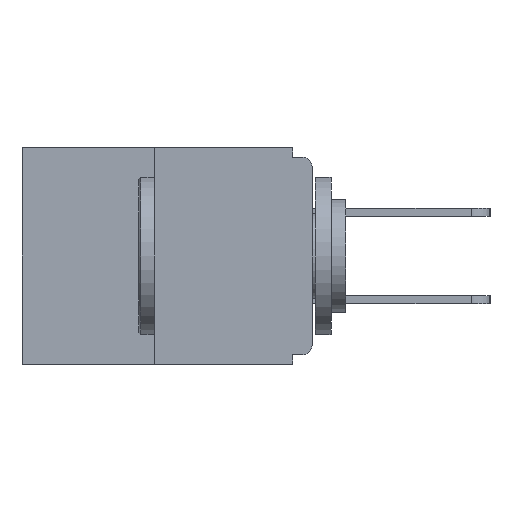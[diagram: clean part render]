
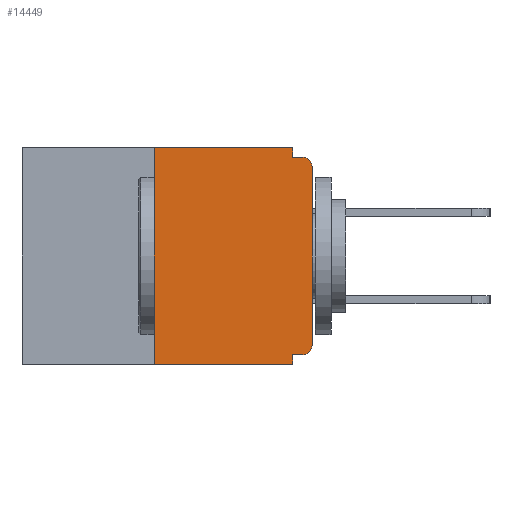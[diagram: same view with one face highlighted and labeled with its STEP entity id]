
A CAD part, left-side view. The second image highlights one B-rep face of the part: STEP entity #14449.
In plain terms, the highlighted planar face has unit normal (-1, 0, 0).
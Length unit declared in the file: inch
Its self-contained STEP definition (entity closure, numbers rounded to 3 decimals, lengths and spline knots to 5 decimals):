
#1213 = DIRECTION ( 'NONE',  ( 0., 0., -1. ) ) ;
#1293 = ORIENTED_EDGE ( 'NONE', *, *, #26827, .T. ) ;
#1649 = LINE ( 'NONE', #18349, #19434 ) ;
#1772 = CARTESIAN_POINT ( 'NONE',  ( 0., 0., -0.313 ) ) ;
#2065 = ORIENTED_EDGE ( 'NONE', *, *, #16569, .T. ) ;
#2437 = VERTEX_POINT ( 'NONE', #18296 ) ;
#2688 = VERTEX_POINT ( 'NONE', #1772 ) ;
#3040 = ORIENTED_EDGE ( 'NONE', *, *, #24897, .T. ) ;
#3080 = CARTESIAN_POINT ( 'NONE',  ( 0., 0., -0.015 ) ) ;
#3087 = ORIENTED_EDGE ( 'NONE', *, *, #24577, .F. ) ;
#3445 = VERTEX_POINT ( 'NONE', #12767 ) ;
#3453 = DIRECTION ( 'NONE',  ( 0., -1., 0. ) ) ;
#4231 = CARTESIAN_POINT ( 'NONE',  ( 0., 0.25, 0. ) ) ;
#4738 = CIRCLE ( 'NONE', #22174, 0.015 ) ;
#5225 = VECTOR ( 'NONE', #21056, 39.37008 ) ;
#5918 = DIRECTION ( 'NONE',  ( 0., 0., 1. ) ) ;
#6887 = DIRECTION ( 'NONE',  ( 0., 0., -1. ) ) ;
#7381 = AXIS2_PLACEMENT_3D ( 'NONE', #15510, #19994, #6887 ) ;
#7421 = CARTESIAN_POINT ( 'NONE',  ( 0., 0.25, -0.343 ) ) ;
#7427 = LINE ( 'NONE', #14130, #16721 ) ;
#7501 = EDGE_CURVE ( 'NONE', #11751, #8629, #21287, .T. ) ;
#7708 = DIRECTION ( 'NONE',  ( 0., 1., 0. ) ) ;
#8007 = EDGE_CURVE ( 'NONE', #20394, #11751, #28143, .T. ) ;
#8028 = VERTEX_POINT ( 'NONE', #23538 ) ;
#8281 = LINE ( 'NONE', #24374, #10684 ) ;
#8629 = VERTEX_POINT ( 'NONE', #19067 ) ;
#8631 = CARTESIAN_POINT ( 'NONE',  ( 0., 0.031, 0. ) ) ;
#9191 = VERTEX_POINT ( 'NONE', #15199 ) ;
#9942 = EDGE_CURVE ( 'NONE', #8028, #9191, #1649, .T. ) ;
#10440 = DIRECTION ( 'NONE',  ( 0., 0., -1. ) ) ;
#10616 = FACE_OUTER_BOUND ( 'NONE', #19601, .T. ) ;
#10684 = VECTOR ( 'NONE', #17773, 39.37008 ) ;
#11025 = ORIENTED_EDGE ( 'NONE', *, *, #12211, .F. ) ;
#11477 = EDGE_CURVE ( 'NONE', #2437, #20394, #26867, .T. ) ;
#11751 = VERTEX_POINT ( 'NONE', #15327 ) ;
#12211 = EDGE_CURVE ( 'NONE', #14949, #2437, #26182, .T. ) ;
#12767 = CARTESIAN_POINT ( 'NONE',  ( 0., 0., -0.03 ) ) ;
#13080 = LINE ( 'NONE', #20679, #15150 ) ;
#13696 = AXIS2_PLACEMENT_3D ( 'NONE', #27669, #25569, #10440 ) ;
#14022 = VECTOR ( 'NONE', #15320, 39.37008 ) ;
#14130 = CARTESIAN_POINT ( 'NONE',  ( 0., 0., 0. ) ) ;
#14449 = ADVANCED_FACE ( 'NONE', ( #10616 ), #25957, .F. ) ;
#14620 = VERTEX_POINT ( 'NONE', #17353 ) ;
#14949 = VERTEX_POINT ( 'NONE', #7421 ) ;
#15150 = VECTOR ( 'NONE', #1213, 39.37008 ) ;
#15199 = CARTESIAN_POINT ( 'NONE',  ( 0., 0.031, -0.328 ) ) ;
#15320 = DIRECTION ( 'NONE',  ( 0., 0., -1. ) ) ;
#15327 = CARTESIAN_POINT ( 'NONE',  ( 0., 0.031, -0.015 ) ) ;
#15460 = VECTOR ( 'NONE', #24614, 39.37008 ) ;
#15510 = CARTESIAN_POINT ( 'NONE',  ( 0., 0.015, -0.313 ) ) ;
#16569 = EDGE_CURVE ( 'NONE', #2688, #3445, #7427, .T. ) ;
#16721 = VECTOR ( 'NONE', #5918, 39.37008 ) ;
#16886 = ORIENTED_EDGE ( 'NONE', *, *, #8007, .F. ) ;
#17353 = CARTESIAN_POINT ( 'NONE',  ( 0., 0.031, -0.343 ) ) ;
#17516 = CARTESIAN_POINT ( 'NONE',  ( 0., 0.015, -0.03 ) ) ;
#17773 = DIRECTION ( 'NONE',  ( 0., -1., 0. ) ) ;
#18061 = CIRCLE ( 'NONE', #7381, 0.015 ) ;
#18296 = CARTESIAN_POINT ( 'NONE',  ( 0., 0.25, 0. ) ) ;
#18349 = CARTESIAN_POINT ( 'NONE',  ( 0., 0., -0.328 ) ) ;
#18773 = CARTESIAN_POINT ( 'NONE',  ( 0., 0.46, 0. ) ) ;
#19067 = CARTESIAN_POINT ( 'NONE',  ( 0., 0.015, -0.015 ) ) ;
#19434 = VECTOR ( 'NONE', #7708, 39.37008 ) ;
#19601 = EDGE_LOOP ( 'NONE', ( #20985, #11025, #3040, #3087, #23898, #1293, #2065, #25624, #22955, #16886 ) ) ;
#19994 = DIRECTION ( 'NONE',  ( -1., 0., 0. ) ) ;
#20394 = VERTEX_POINT ( 'NONE', #27845 ) ;
#20516 = EDGE_CURVE ( 'NONE', #3445, #8629, #4738, .T. ) ;
#20679 = CARTESIAN_POINT ( 'NONE',  ( 0., 0.031, -0.343 ) ) ;
#20695 = VECTOR ( 'NONE', #3453, 39.37008 ) ;
#20985 = ORIENTED_EDGE ( 'NONE', *, *, #11477, .F. ) ;
#21056 = DIRECTION ( 'NONE',  ( 0., 0., 1. ) ) ;
#21287 = LINE ( 'NONE', #3080, #15460 ) ;
#22174 = AXIS2_PLACEMENT_3D ( 'NONE', #17516, #24022, #23847 ) ;
#22955 = ORIENTED_EDGE ( 'NONE', *, *, #7501, .F. ) ;
#23538 = CARTESIAN_POINT ( 'NONE',  ( 0., 0.015, -0.328 ) ) ;
#23847 = DIRECTION ( 'NONE',  ( 0., 0., -1. ) ) ;
#23898 = ORIENTED_EDGE ( 'NONE', *, *, #9942, .F. ) ;
#24022 = DIRECTION ( 'NONE',  ( -1., 0., 0. ) ) ;
#24374 = CARTESIAN_POINT ( 'NONE',  ( 0., 0.46, -0.343 ) ) ;
#24577 = EDGE_CURVE ( 'NONE', #9191, #14620, #13080, .T. ) ;
#24614 = DIRECTION ( 'NONE',  ( 0., -1., 0. ) ) ;
#24897 = EDGE_CURVE ( 'NONE', #14949, #14620, #8281, .T. ) ;
#25569 = DIRECTION ( 'NONE',  ( 1., 0., 0. ) ) ;
#25624 = ORIENTED_EDGE ( 'NONE', *, *, #20516, .T. ) ;
#25957 = PLANE ( 'NONE',  #13696 ) ;
#26182 = LINE ( 'NONE', #4231, #5225 ) ;
#26827 = EDGE_CURVE ( 'NONE', #8028, #2688, #18061, .T. ) ;
#26867 = LINE ( 'NONE', #18773, #20695 ) ;
#27669 = CARTESIAN_POINT ( 'NONE',  ( 0., 0.46, 0. ) ) ;
#27845 = CARTESIAN_POINT ( 'NONE',  ( 0., 0.031, 0. ) ) ;
#28143 = LINE ( 'NONE', #8631, #14022 ) ;
